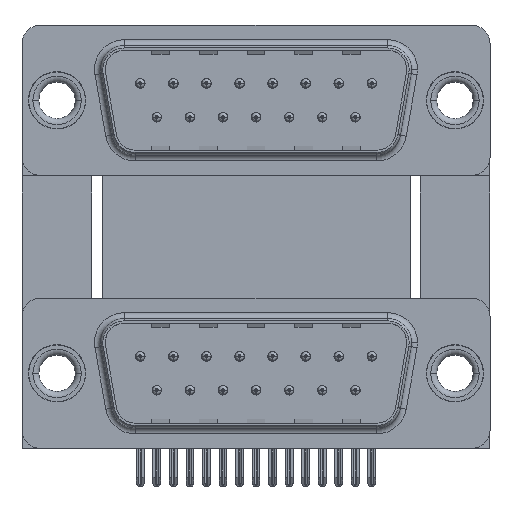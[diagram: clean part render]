
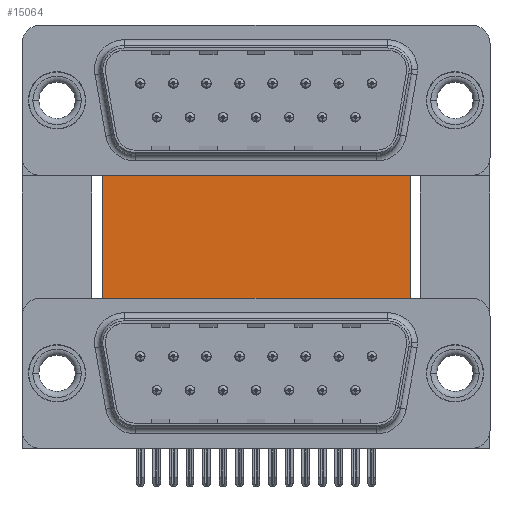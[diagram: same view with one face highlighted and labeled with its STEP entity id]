
A CAD part, top view. The second image highlights one B-rep face of the part: STEP entity #15064.
In plain terms, the highlighted planar face has unit normal (0, 0, 1).
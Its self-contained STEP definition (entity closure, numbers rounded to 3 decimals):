
#296 = EDGE_LOOP ( 'NONE', ( #10923, #17674, #26333, #12083 ) ) ;
#472 = CARTESIAN_POINT ( 'NONE',  ( 3.79, 16.585, -12. ) ) ;
#1338 = VERTEX_POINT ( 'NONE', #5303 ) ;
#1351 = EDGE_CURVE ( 'NONE', #7174, #27148, #25350, .T. ) ;
#2638 = CARTESIAN_POINT ( 'NONE',  ( 3.79, -3.735, -12. ) ) ;
#5303 = CARTESIAN_POINT ( 'NONE',  ( 29.58, 16.585, -12. ) ) ;
#7154 = DIRECTION ( 'NONE',  ( -1., 0., 0. ) ) ;
#7174 = VERTEX_POINT ( 'NONE', #20420 ) ;
#9717 = DIRECTION ( 'NONE',  ( 1., 0., 0. ) ) ;
#10034 = EDGE_CURVE ( 'NONE', #1338, #27148, #22152, .T. ) ;
#10923 = ORIENTED_EDGE ( 'NONE', *, *, #1351, .T. ) ;
#11037 = VECTOR ( 'NONE', #9717, 1000. ) ;
#11275 = PLANE ( 'NONE',  #28911 ) ;
#11808 = LINE ( 'NONE', #14158, #22520 ) ;
#12083 = ORIENTED_EDGE ( 'NONE', *, *, #26885, .T. ) ;
#14158 = CARTESIAN_POINT ( 'NONE',  ( 3.79, 16.585, -12. ) ) ;
#15064 = ADVANCED_FACE ( 'NONE', ( #24999 ), #11275, .F. ) ;
#15452 = CARTESIAN_POINT ( 'NONE',  ( 29.58, 16.585, -12. ) ) ;
#15673 = CARTESIAN_POINT ( 'NONE',  ( 3.79, 16.585, -12. ) ) ;
#16094 = DIRECTION ( 'NONE',  ( 0., 0., -1. ) ) ;
#17674 = ORIENTED_EDGE ( 'NONE', *, *, #10034, .F. ) ;
#17904 = VECTOR ( 'NONE', #23294, 1000. ) ;
#20420 = CARTESIAN_POINT ( 'NONE',  ( 3.79, -3.735, -12. ) ) ;
#22152 = LINE ( 'NONE', #15452, #22219 ) ;
#22219 = VECTOR ( 'NONE', #26418, 1000. ) ;
#22520 = VECTOR ( 'NONE', #27302, 1000. ) ;
#23293 = VERTEX_POINT ( 'NONE', #472 ) ;
#23294 = DIRECTION ( 'NONE',  ( 0., -1., 0. ) ) ;
#24631 = EDGE_CURVE ( 'NONE', #23293, #1338, #11808, .T. ) ;
#24999 = FACE_OUTER_BOUND ( 'NONE', #296, .T. ) ;
#25350 = LINE ( 'NONE', #2638, #11037 ) ;
#25570 = CARTESIAN_POINT ( 'NONE',  ( 29.58, -3.735, -12. ) ) ;
#25768 = CARTESIAN_POINT ( 'NONE',  ( 3.79, 16.585, -12. ) ) ;
#25919 = LINE ( 'NONE', #25768, #17904 ) ;
#26333 = ORIENTED_EDGE ( 'NONE', *, *, #24631, .F. ) ;
#26418 = DIRECTION ( 'NONE',  ( 0., -1., 0. ) ) ;
#26885 = EDGE_CURVE ( 'NONE', #23293, #7174, #25919, .T. ) ;
#27148 = VERTEX_POINT ( 'NONE', #25570 ) ;
#27302 = DIRECTION ( 'NONE',  ( 1., 0., 0. ) ) ;
#28911 = AXIS2_PLACEMENT_3D ( 'NONE', #15673, #16094, #7154 ) ;
